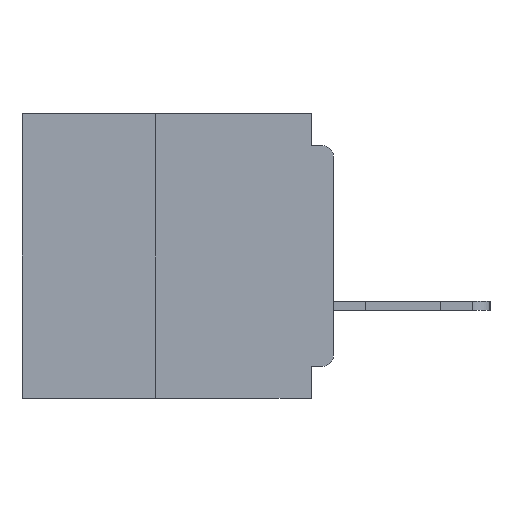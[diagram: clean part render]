
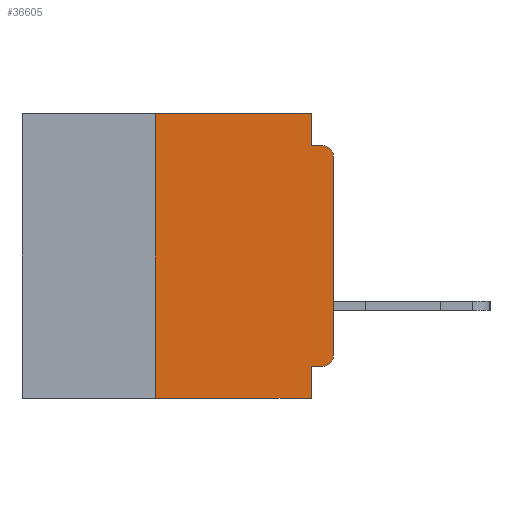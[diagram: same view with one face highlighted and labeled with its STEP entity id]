
A CAD part, left-side view. The second image highlights one B-rep face of the part: STEP entity #36605.
In plain terms, the highlighted planar face has unit normal (-1, 0, 0).
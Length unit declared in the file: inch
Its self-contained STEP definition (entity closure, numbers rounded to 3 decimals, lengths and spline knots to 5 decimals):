
#196 = EDGE_CURVE ( 'NONE', #34068, #4379, #32147, .T. ) ;
#937 = LINE ( 'NONE', #41831, #37116 ) ;
#1824 = VECTOR ( 'NONE', #40148, 39.37008 ) ;
#2159 = ORIENTED_EDGE ( 'NONE', *, *, #24018, .T. ) ;
#2913 = LINE ( 'NONE', #36663, #1824 ) ;
#2964 = DIRECTION ( 'NONE',  ( 0., 0., 1. ) ) ;
#3268 = CIRCLE ( 'NONE', #27337, 0.015 ) ;
#3973 = ORIENTED_EDGE ( 'NONE', *, *, #39473, .F. ) ;
#4203 = VECTOR ( 'NONE', #20049, 39.37008 ) ;
#4379 = VERTEX_POINT ( 'NONE', #31122 ) ;
#6184 = CARTESIAN_POINT ( 'NONE',  ( 0., 0.25, -0.4 ) ) ;
#6276 = LINE ( 'NONE', #16202, #23773 ) ;
#6408 = ORIENTED_EDGE ( 'NONE', *, *, #18804, .F. ) ;
#6907 = CARTESIAN_POINT ( 'NONE',  ( 0., 0.437, 0. ) ) ;
#7536 = AXIS2_PLACEMENT_3D ( 'NONE', #6907, #10419, #34872 ) ;
#8131 = EDGE_CURVE ( 'NONE', #18702, #31968, #9146, .T. ) ;
#8812 = LINE ( 'NONE', #30514, #18122 ) ;
#8925 = CARTESIAN_POINT ( 'NONE',  ( 0., 0., -0.06 ) ) ;
#9146 = CIRCLE ( 'NONE', #32618, 0.015 ) ;
#9407 = CARTESIAN_POINT ( 'NONE',  ( 0., 0.031, 0. ) ) ;
#9619 = EDGE_CURVE ( 'NONE', #14901, #18702, #39429, .T. ) ;
#10419 = DIRECTION ( 'NONE',  ( 1., 0., 0. ) ) ;
#10714 = ORIENTED_EDGE ( 'NONE', *, *, #9619, .T. ) ;
#11207 = ORIENTED_EDGE ( 'NONE', *, *, #37363, .T. ) ;
#11577 = CARTESIAN_POINT ( 'NONE',  ( 0., 0.437, 0. ) ) ;
#12327 = ORIENTED_EDGE ( 'NONE', *, *, #8131, .T. ) ;
#14111 = EDGE_CURVE ( 'NONE', #42201, #40058, #6276, .T. ) ;
#14901 = VERTEX_POINT ( 'NONE', #17208 ) ;
#15018 = DIRECTION ( 'NONE',  ( -1., 0., 0. ) ) ;
#16202 = CARTESIAN_POINT ( 'NONE',  ( 0., 0.25, -0.4 ) ) ;
#17208 = CARTESIAN_POINT ( 'NONE',  ( 0., 0., -0.34 ) ) ;
#17546 = EDGE_CURVE ( 'NONE', #21049, #41265, #25376, .T. ) ;
#18122 = VECTOR ( 'NONE', #34013, 39.37008 ) ;
#18135 = CARTESIAN_POINT ( 'NONE',  ( 0., 0.25, 0. ) ) ;
#18702 = VERTEX_POINT ( 'NONE', #8925 ) ;
#18804 = EDGE_CURVE ( 'NONE', #4379, #31968, #8812, .T. ) ;
#18813 = CARTESIAN_POINT ( 'NONE',  ( 0., 0.015, -0.34 ) ) ;
#19759 = DIRECTION ( 'NONE',  ( 0., 0., 1. ) ) ;
#20049 = DIRECTION ( 'NONE',  ( 0., 0., -1. ) ) ;
#20869 = VECTOR ( 'NONE', #2964, 39.37008 ) ;
#21049 = VERTEX_POINT ( 'NONE', #37985 ) ;
#21567 = CARTESIAN_POINT ( 'NONE',  ( 0., 0.031, -0.355 ) ) ;
#21600 = CARTESIAN_POINT ( 'NONE',  ( 0., 0.031, 0. ) ) ;
#22308 = DIRECTION ( 'NONE',  ( 0., 0., -1. ) ) ;
#23699 = CARTESIAN_POINT ( 'NONE',  ( 0., 0., -0.355 ) ) ;
#23773 = VECTOR ( 'NONE', #19759, 39.37008 ) ;
#24018 = EDGE_CURVE ( 'NONE', #21049, #14901, #3268, .T. ) ;
#24588 = FACE_OUTER_BOUND ( 'NONE', #29367, .T. ) ;
#25376 = LINE ( 'NONE', #23699, #34657 ) ;
#26022 = VERTEX_POINT ( 'NONE', #28719 ) ;
#26076 = EDGE_CURVE ( 'NONE', #40058, #34068, #35390, .T. ) ;
#27337 = AXIS2_PLACEMENT_3D ( 'NONE', #18813, #43194, #22308 ) ;
#27973 = DIRECTION ( 'NONE',  ( 0., -1., 0. ) ) ;
#28719 = CARTESIAN_POINT ( 'NONE',  ( 0., 0.031, -0.4 ) ) ;
#29178 = DIRECTION ( 'NONE',  ( 0., -1., 0. ) ) ;
#29367 = EDGE_LOOP ( 'NONE', ( #10714, #12327, #6408, #31971, #32451, #30750, #11207, #3973, #31738, #2159 ) ) ;
#30514 = CARTESIAN_POINT ( 'NONE',  ( 0., 0., -0.045 ) ) ;
#30750 = ORIENTED_EDGE ( 'NONE', *, *, #14111, .F. ) ;
#31122 = CARTESIAN_POINT ( 'NONE',  ( 0., 0.031, -0.045 ) ) ;
#31372 = PLANE ( 'NONE',  #7536 ) ;
#31738 = ORIENTED_EDGE ( 'NONE', *, *, #17546, .F. ) ;
#31968 = VERTEX_POINT ( 'NONE', #39674 ) ;
#31971 = ORIENTED_EDGE ( 'NONE', *, *, #196, .F. ) ;
#32147 = LINE ( 'NONE', #21600, #4203 ) ;
#32451 = ORIENTED_EDGE ( 'NONE', *, *, #26076, .F. ) ;
#32618 = AXIS2_PLACEMENT_3D ( 'NONE', #35998, #15018, #39451 ) ;
#34013 = DIRECTION ( 'NONE',  ( 0., -1., 0. ) ) ;
#34068 = VERTEX_POINT ( 'NONE', #9407 ) ;
#34300 = VECTOR ( 'NONE', #29178, 39.37008 ) ;
#34657 = VECTOR ( 'NONE', #44560, 39.37008 ) ;
#34872 = DIRECTION ( 'NONE',  ( 0., 0., -1. ) ) ;
#35390 = LINE ( 'NONE', #11577, #34300 ) ;
#35998 = CARTESIAN_POINT ( 'NONE',  ( 0., 0.015, -0.06 ) ) ;
#36605 = ADVANCED_FACE ( 'NONE', ( #24588 ), #31372, .F. ) ;
#36663 = CARTESIAN_POINT ( 'NONE',  ( 0., 0.031, -0.4 ) ) ;
#37116 = VECTOR ( 'NONE', #27973, 39.37008 ) ;
#37363 = EDGE_CURVE ( 'NONE', #42201, #26022, #937, .T. ) ;
#37985 = CARTESIAN_POINT ( 'NONE',  ( 0., 0.015, -0.355 ) ) ;
#39429 = LINE ( 'NONE', #44830, #20869 ) ;
#39451 = DIRECTION ( 'NONE',  ( 0., 0., -1. ) ) ;
#39473 = EDGE_CURVE ( 'NONE', #41265, #26022, #2913, .T. ) ;
#39674 = CARTESIAN_POINT ( 'NONE',  ( 0., 0.015, -0.045 ) ) ;
#40058 = VERTEX_POINT ( 'NONE', #18135 ) ;
#40148 = DIRECTION ( 'NONE',  ( 0., 0., -1. ) ) ;
#41265 = VERTEX_POINT ( 'NONE', #21567 ) ;
#41831 = CARTESIAN_POINT ( 'NONE',  ( 0., 0.437, -0.4 ) ) ;
#42201 = VERTEX_POINT ( 'NONE', #6184 ) ;
#43194 = DIRECTION ( 'NONE',  ( -1., 0., 0. ) ) ;
#44560 = DIRECTION ( 'NONE',  ( 0., 1., 0. ) ) ;
#44830 = CARTESIAN_POINT ( 'NONE',  ( 0., 0., 0. ) ) ;
